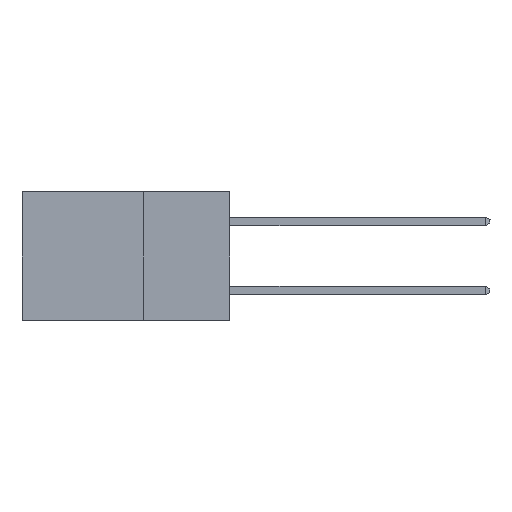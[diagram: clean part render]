
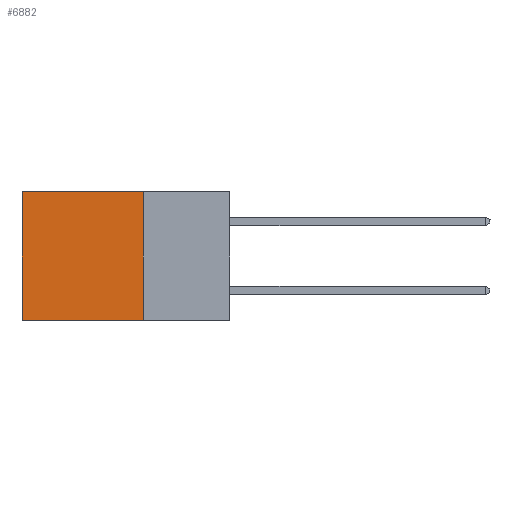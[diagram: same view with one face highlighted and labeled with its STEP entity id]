
A CAD part, left-side view. The second image highlights one B-rep face of the part: STEP entity #6882.
In plain terms, the highlighted planar face has unit normal (-1, 0, 0).
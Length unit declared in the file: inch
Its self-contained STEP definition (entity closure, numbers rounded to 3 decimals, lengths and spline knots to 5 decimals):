
#415 = DIRECTION ( 'NONE',  ( 0., 0., -1. ) ) ;
#1109 = DIRECTION ( 'NONE',  ( 0., 0., -1. ) ) ;
#1117 = VECTOR ( 'NONE', #13007, 39.37008 ) ;
#2483 = CARTESIAN_POINT ( 'NONE',  ( 0.2615, 0.25, 0. ) ) ;
#3171 = EDGE_CURVE ( 'NONE', #10176, #12121, #16626, .T. ) ;
#3300 = CARTESIAN_POINT ( 'NONE',  ( 0.2615, 0.6, -0.37 ) ) ;
#3744 = CARTESIAN_POINT ( 'NONE',  ( 0.2615, 0.6, 0. ) ) ;
#5748 = DIRECTION ( 'NONE',  ( 1., 0., 0. ) ) ;
#6650 = EDGE_CURVE ( 'NONE', #12121, #10431, #19169, .T. ) ;
#6882 = ADVANCED_FACE ( 'NONE', ( #15117 ), #12152, .F. ) ;
#7646 = VECTOR ( 'NONE', #9411, 39.37008 ) ;
#8932 = CARTESIAN_POINT ( 'NONE',  ( 0.2615, 0.25, 0. ) ) ;
#8987 = ORIENTED_EDGE ( 'NONE', *, *, #3171, .T. ) ;
#9411 = DIRECTION ( 'NONE',  ( 0., 1., 0. ) ) ;
#9691 = ORIENTED_EDGE ( 'NONE', *, *, #16863, .F. ) ;
#10176 = VERTEX_POINT ( 'NONE', #8932 ) ;
#10431 = VERTEX_POINT ( 'NONE', #13140 ) ;
#10865 = VERTEX_POINT ( 'NONE', #14449 ) ;
#11367 = VECTOR ( 'NONE', #415, 39.37008 ) ;
#11718 = EDGE_LOOP ( 'NONE', ( #15190, #9691, #12376, #8987 ) ) ;
#11728 = AXIS2_PLACEMENT_3D ( 'NONE', #19864, #5748, #1109 ) ;
#12121 = VERTEX_POINT ( 'NONE', #3744 ) ;
#12152 = PLANE ( 'NONE',  #11728 ) ;
#12376 = ORIENTED_EDGE ( 'NONE', *, *, #14438, .F. ) ;
#13007 = DIRECTION ( 'NONE',  ( 0., 1., 0. ) ) ;
#13140 = CARTESIAN_POINT ( 'NONE',  ( 0.2615, 0.6, -0.37 ) ) ;
#13272 = LINE ( 'NONE', #19764, #17142 ) ;
#14438 = EDGE_CURVE ( 'NONE', #10176, #10865, #13272, .T. ) ;
#14449 = CARTESIAN_POINT ( 'NONE',  ( 0.2615, 0.25, -0.37 ) ) ;
#15117 = FACE_OUTER_BOUND ( 'NONE', #11718, .T. ) ;
#15190 = ORIENTED_EDGE ( 'NONE', *, *, #6650, .T. ) ;
#16626 = LINE ( 'NONE', #2483, #1117 ) ;
#16693 = DIRECTION ( 'NONE',  ( 0., 0., -1. ) ) ;
#16863 = EDGE_CURVE ( 'NONE', #10865, #10431, #18884, .T. ) ;
#17142 = VECTOR ( 'NONE', #16693, 39.37008 ) ;
#18787 = CARTESIAN_POINT ( 'NONE',  ( 0.2615, 0.25, -0.37 ) ) ;
#18884 = LINE ( 'NONE', #18787, #7646 ) ;
#19169 = LINE ( 'NONE', #3300, #11367 ) ;
#19764 = CARTESIAN_POINT ( 'NONE',  ( 0.2615, 0.25, -0.37 ) ) ;
#19864 = CARTESIAN_POINT ( 'NONE',  ( 0.2615, 0.25, -0.37 ) ) ;
